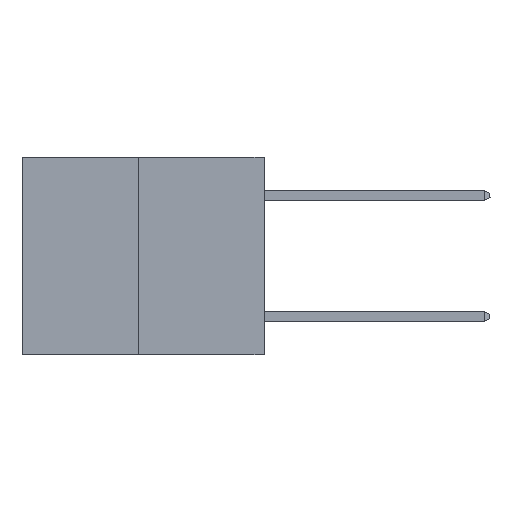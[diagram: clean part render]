
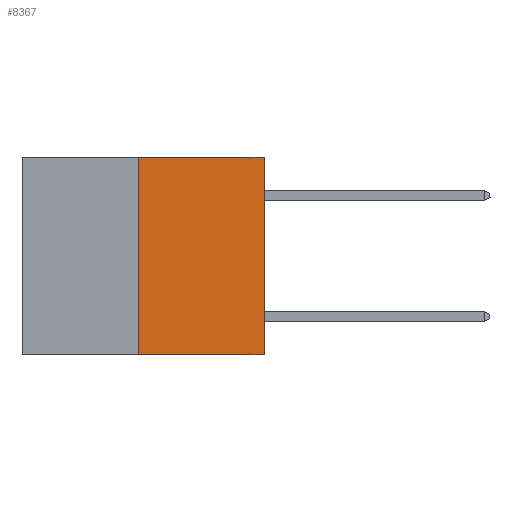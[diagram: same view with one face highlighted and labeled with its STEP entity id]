
A CAD part, left-side view. The second image highlights one B-rep face of the part: STEP entity #8367.
In plain terms, the highlighted planar face has unit normal (-1, 0, 0).
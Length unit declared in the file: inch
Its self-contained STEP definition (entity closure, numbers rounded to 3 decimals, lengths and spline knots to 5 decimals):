
#594 = EDGE_CURVE ( 'NONE', #4165, #2931, #10015, .T. ) ;
#640 = FACE_OUTER_BOUND ( 'NONE', #17878, .T. ) ;
#1296 = CARTESIAN_POINT ( 'NONE',  ( 0., 0., -0.49 ) ) ;
#2931 = VERTEX_POINT ( 'NONE', #1296 ) ;
#3265 = CARTESIAN_POINT ( 'NONE',  ( 0., 0.6, 0. ) ) ;
#3609 = CARTESIAN_POINT ( 'NONE',  ( 0., 0.312, 0. ) ) ;
#4165 = VERTEX_POINT ( 'NONE', #17690 ) ;
#4404 = CARTESIAN_POINT ( 'NONE',  ( 0., 0., 0. ) ) ;
#4466 = VERTEX_POINT ( 'NONE', #3609 ) ;
#5605 = EDGE_CURVE ( 'NONE', #4165, #4466, #20164, .T. ) ;
#6563 = EDGE_CURVE ( 'NONE', #2931, #7407, #11318, .T. ) ;
#7407 = VERTEX_POINT ( 'NONE', #10352 ) ;
#7793 = ORIENTED_EDGE ( 'NONE', *, *, #594, .T. ) ;
#7888 = DIRECTION ( 'NONE',  ( 0., 0., -1. ) ) ;
#8367 = ADVANCED_FACE ( 'NONE', ( #640 ), #21743, .F. ) ;
#10015 = LINE ( 'NONE', #15088, #21000 ) ;
#10352 = CARTESIAN_POINT ( 'NONE',  ( 0., 0., 0. ) ) ;
#10935 = DIRECTION ( 'NONE',  ( 0., -1., 0. ) ) ;
#10959 = AXIS2_PLACEMENT_3D ( 'NONE', #12880, #16325, #7888 ) ;
#11318 = LINE ( 'NONE', #4404, #22564 ) ;
#12829 = ORIENTED_EDGE ( 'NONE', *, *, #6563, .T. ) ;
#12880 = CARTESIAN_POINT ( 'NONE',  ( 0., 0.6, 0. ) ) ;
#12964 = DIRECTION ( 'NONE',  ( 0., 0., 1. ) ) ;
#13184 = EDGE_CURVE ( 'NONE', #4466, #7407, #21835, .T. ) ;
#15088 = CARTESIAN_POINT ( 'NONE',  ( 0., 0.6, -0.49 ) ) ;
#15520 = VECTOR ( 'NONE', #18948, 39.37008 ) ;
#16325 = DIRECTION ( 'NONE',  ( 1., 0., 0. ) ) ;
#17457 = VECTOR ( 'NONE', #20747, 39.37008 ) ;
#17573 = ORIENTED_EDGE ( 'NONE', *, *, #13184, .F. ) ;
#17690 = CARTESIAN_POINT ( 'NONE',  ( 0., 0.312, -0.49 ) ) ;
#17878 = EDGE_LOOP ( 'NONE', ( #19552, #7793, #12829, #17573 ) ) ;
#18948 = DIRECTION ( 'NONE',  ( 0., 0., 1. ) ) ;
#19104 = CARTESIAN_POINT ( 'NONE',  ( 0., 0.312, -0.49 ) ) ;
#19552 = ORIENTED_EDGE ( 'NONE', *, *, #5605, .F. ) ;
#20164 = LINE ( 'NONE', #19104, #15520 ) ;
#20747 = DIRECTION ( 'NONE',  ( 0., -1., 0. ) ) ;
#21000 = VECTOR ( 'NONE', #10935, 39.37008 ) ;
#21743 = PLANE ( 'NONE',  #10959 ) ;
#21835 = LINE ( 'NONE', #3265, #17457 ) ;
#22564 = VECTOR ( 'NONE', #12964, 39.37008 ) ;
